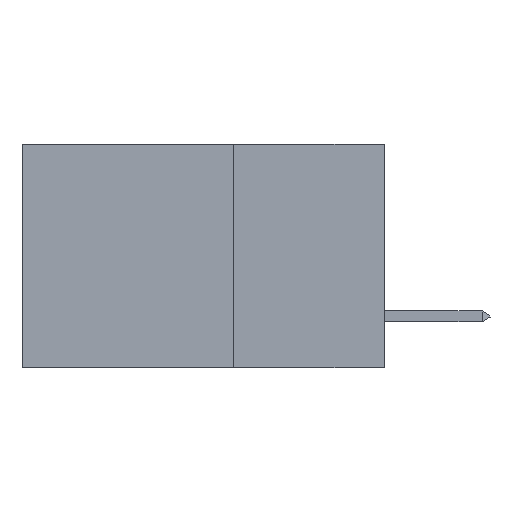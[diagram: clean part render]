
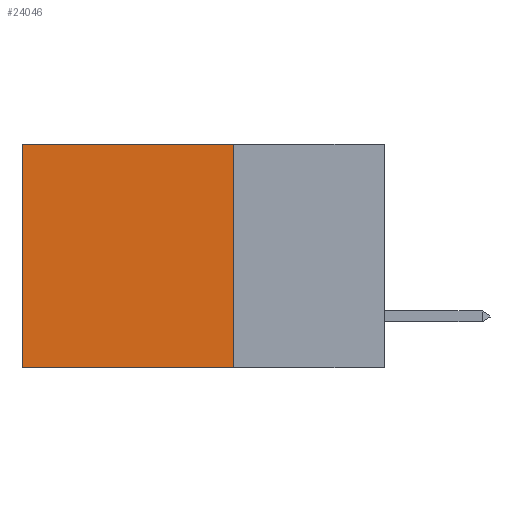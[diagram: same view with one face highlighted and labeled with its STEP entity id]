
A CAD part, left-side view. The second image highlights one B-rep face of the part: STEP entity #24046.
In plain terms, the highlighted planar face has unit normal (-1, 0, 0).
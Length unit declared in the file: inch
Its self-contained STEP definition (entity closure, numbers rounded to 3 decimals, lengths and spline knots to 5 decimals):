
#867 = CARTESIAN_POINT ( 'NONE',  ( 0.2875, 0.6, 0. ) ) ;
#1975 = LINE ( 'NONE', #42849, #4379 ) ;
#2083 = LINE ( 'NONE', #42482, #39099 ) ;
#3695 = ORIENTED_EDGE ( 'NONE', *, *, #37172, .T. ) ;
#3857 = LINE ( 'NONE', #31954, #22011 ) ;
#4379 = VECTOR ( 'NONE', #38592, 39.37008 ) ;
#5343 = DIRECTION ( 'NONE',  ( 0., 0., -1. ) ) ;
#6564 = CARTESIAN_POINT ( 'NONE',  ( 0.2875, 0.6, 0. ) ) ;
#7800 = EDGE_LOOP ( 'NONE', ( #3695, #16267, #12881, #22695 ) ) ;
#9573 = CARTESIAN_POINT ( 'NONE',  ( 0.2875, 0.25, 0. ) ) ;
#10453 = CARTESIAN_POINT ( 'NONE',  ( 0.2875, 0.6, -0.37 ) ) ;
#10487 = FACE_OUTER_BOUND ( 'NONE', #7800, .T. ) ;
#12881 = ORIENTED_EDGE ( 'NONE', *, *, #23968, .F. ) ;
#15115 = VERTEX_POINT ( 'NONE', #6564 ) ;
#15175 = DIRECTION ( 'NONE',  ( 0., 1., 0. ) ) ;
#16267 = ORIENTED_EDGE ( 'NONE', *, *, #17472, .F. ) ;
#16808 = VERTEX_POINT ( 'NONE', #10453 ) ;
#17472 = EDGE_CURVE ( 'NONE', #25908, #16808, #2083, .T. ) ;
#17983 = AXIS2_PLACEMENT_3D ( 'NONE', #9573, #25155, #32630 ) ;
#22011 = VECTOR ( 'NONE', #5343, 39.37008 ) ;
#22695 = ORIENTED_EDGE ( 'NONE', *, *, #35605, .T. ) ;
#23968 = EDGE_CURVE ( 'NONE', #46205, #25908, #3857, .T. ) ;
#24046 = ADVANCED_FACE ( 'NONE', ( #10487 ), #33130, .F. ) ;
#25155 = DIRECTION ( 'NONE',  ( 1., 0., 0. ) ) ;
#25908 = VERTEX_POINT ( 'NONE', #31830 ) ;
#31830 = CARTESIAN_POINT ( 'NONE',  ( 0.2875, 0.25, -0.37 ) ) ;
#31954 = CARTESIAN_POINT ( 'NONE',  ( 0.2875, 0.25, 0. ) ) ;
#32630 = DIRECTION ( 'NONE',  ( 0., 0., -1. ) ) ;
#33130 = PLANE ( 'NONE',  #17983 ) ;
#34537 = VECTOR ( 'NONE', #36607, 39.37008 ) ;
#35605 = EDGE_CURVE ( 'NONE', #46205, #15115, #1975, .T. ) ;
#35708 = CARTESIAN_POINT ( 'NONE',  ( 0.2875, 0.25, 0. ) ) ;
#36607 = DIRECTION ( 'NONE',  ( 0., 0., -1. ) ) ;
#37172 = EDGE_CURVE ( 'NONE', #15115, #16808, #44906, .T. ) ;
#38592 = DIRECTION ( 'NONE',  ( 0., 1., 0. ) ) ;
#39099 = VECTOR ( 'NONE', #15175, 39.37008 ) ;
#42482 = CARTESIAN_POINT ( 'NONE',  ( 0.2875, 0.25, -0.37 ) ) ;
#42849 = CARTESIAN_POINT ( 'NONE',  ( 0.2875, 0.25, 0. ) ) ;
#44906 = LINE ( 'NONE', #867, #34537 ) ;
#46205 = VERTEX_POINT ( 'NONE', #35708 ) ;
